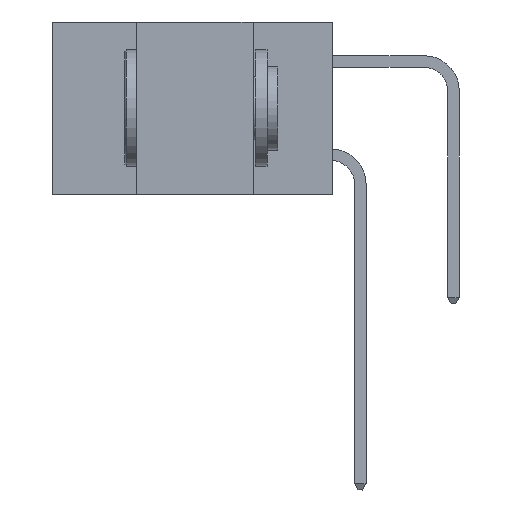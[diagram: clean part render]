
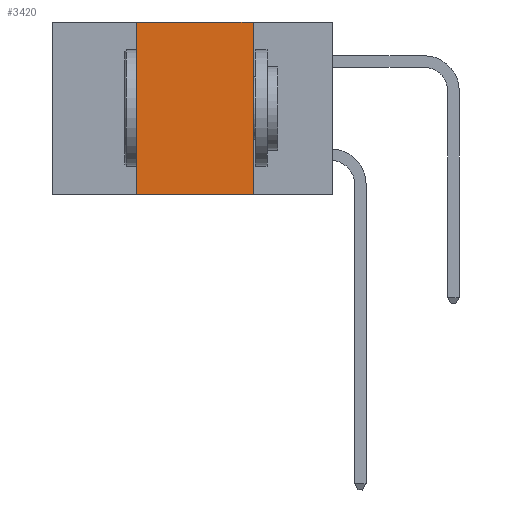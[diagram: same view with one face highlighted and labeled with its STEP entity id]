
A CAD part, left-side view. The second image highlights one B-rep face of the part: STEP entity #3420.
In plain terms, the highlighted planar face has unit normal (-1, 0, 0).
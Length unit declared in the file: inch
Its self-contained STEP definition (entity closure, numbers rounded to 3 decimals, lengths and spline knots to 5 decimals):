
#221 = CARTESIAN_POINT ( 'NONE',  ( 0., 0.6, 0. ) ) ;
#609 = VECTOR ( 'NONE', #3210, 39.37008 ) ;
#1946 = EDGE_CURVE ( 'NONE', #9576, #4088, #18674, .T. ) ;
#1991 = CARTESIAN_POINT ( 'NONE',  ( 0., 0.17, 0. ) ) ;
#2854 = CARTESIAN_POINT ( 'NONE',  ( 0., 0.42, -0.37 ) ) ;
#3210 = DIRECTION ( 'NONE',  ( 0., 0., 1. ) ) ;
#3420 = ADVANCED_FACE ( 'NONE', ( #14396 ), #5704, .F. ) ;
#3515 = DIRECTION ( 'NONE',  ( 0., 0., -1. ) ) ;
#4088 = VERTEX_POINT ( 'NONE', #15962 ) ;
#5563 = DIRECTION ( 'NONE',  ( 0., -1., 0. ) ) ;
#5684 = DIRECTION ( 'NONE',  ( 0., -1., 0. ) ) ;
#5704 = PLANE ( 'NONE',  #9407 ) ;
#6000 = VERTEX_POINT ( 'NONE', #11311 ) ;
#7150 = ORIENTED_EDGE ( 'NONE', *, *, #1946, .F. ) ;
#7317 = VECTOR ( 'NONE', #5563, 39.37008 ) ;
#7826 = VERTEX_POINT ( 'NONE', #21142 ) ;
#7951 = VECTOR ( 'NONE', #5684, 39.37008 ) ;
#9186 = CARTESIAN_POINT ( 'NONE',  ( 0., 0.6, -0.37 ) ) ;
#9407 = AXIS2_PLACEMENT_3D ( 'NONE', #21790, #20237, #3515 ) ;
#9576 = VERTEX_POINT ( 'NONE', #1991 ) ;
#10317 = EDGE_CURVE ( 'NONE', #7826, #4088, #11244, .T. ) ;
#10998 = LINE ( 'NONE', #221, #7951 ) ;
#11244 = LINE ( 'NONE', #9186, #7317 ) ;
#11311 = CARTESIAN_POINT ( 'NONE',  ( 0., 0.42, 0. ) ) ;
#11694 = EDGE_CURVE ( 'NONE', #6000, #9576, #10998, .T. ) ;
#11912 = ORIENTED_EDGE ( 'NONE', *, *, #13314, .F. ) ;
#13314 = EDGE_CURVE ( 'NONE', #7826, #6000, #15908, .T. ) ;
#14396 = FACE_OUTER_BOUND ( 'NONE', #17236, .T. ) ;
#15150 = CARTESIAN_POINT ( 'NONE',  ( 0., 0.17, -0.37 ) ) ;
#15292 = ORIENTED_EDGE ( 'NONE', *, *, #10317, .T. ) ;
#15908 = LINE ( 'NONE', #2854, #609 ) ;
#15962 = CARTESIAN_POINT ( 'NONE',  ( 0., 0.17, -0.37 ) ) ;
#16849 = DIRECTION ( 'NONE',  ( 0., 0., -1. ) ) ;
#17236 = EDGE_LOOP ( 'NONE', ( #7150, #23848, #11912, #15292 ) ) ;
#18674 = LINE ( 'NONE', #15150, #23210 ) ;
#20237 = DIRECTION ( 'NONE',  ( 1., 0., 0. ) ) ;
#21142 = CARTESIAN_POINT ( 'NONE',  ( 0., 0.42, -0.37 ) ) ;
#21790 = CARTESIAN_POINT ( 'NONE',  ( 0., 0.6, 0. ) ) ;
#23210 = VECTOR ( 'NONE', #16849, 39.37008 ) ;
#23848 = ORIENTED_EDGE ( 'NONE', *, *, #11694, .F. ) ;
